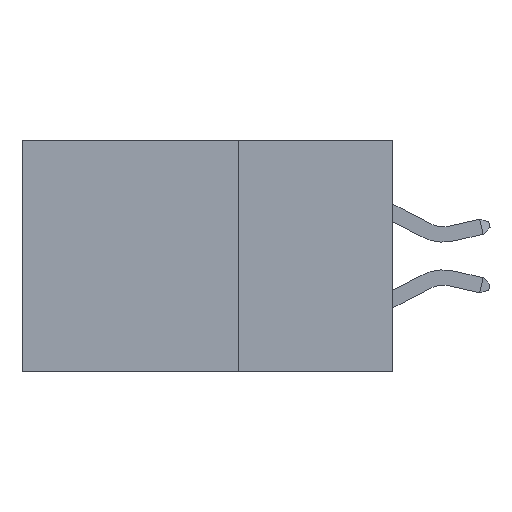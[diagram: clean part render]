
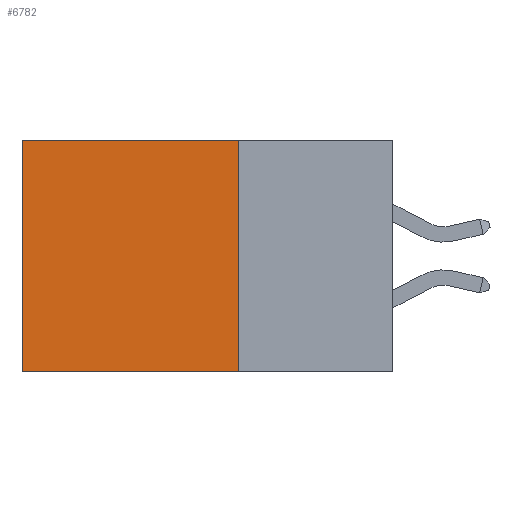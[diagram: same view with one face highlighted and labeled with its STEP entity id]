
A CAD part, left-side view. The second image highlights one B-rep face of the part: STEP entity #6782.
In plain terms, the highlighted planar face has unit normal (-1, 0, 0).
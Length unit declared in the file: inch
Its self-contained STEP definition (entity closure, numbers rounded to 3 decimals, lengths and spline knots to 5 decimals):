
#1126 = LINE ( 'NONE', #19039, #11063 ) ;
#1216 = EDGE_CURVE ( 'NONE', #10784, #21238, #11358, .T. ) ;
#1342 = VERTEX_POINT ( 'NONE', #4020 ) ;
#2004 = CARTESIAN_POINT ( 'NONE',  ( 0.2875, 0.25, -0.375 ) ) ;
#2983 = AXIS2_PLACEMENT_3D ( 'NONE', #11128, #14328, #4358 ) ;
#3239 = CARTESIAN_POINT ( 'NONE',  ( 0.2875, 0.25, 0. ) ) ;
#4020 = CARTESIAN_POINT ( 'NONE',  ( 0.2875, 0.25, 0. ) ) ;
#4358 = DIRECTION ( 'NONE',  ( 0., 0., -1. ) ) ;
#5771 = PLANE ( 'NONE',  #2983 ) ;
#6770 = VECTOR ( 'NONE', #12185, 39.37008 ) ;
#6782 = ADVANCED_FACE ( 'NONE', ( #12135 ), #5771, .F. ) ;
#7370 = DIRECTION ( 'NONE',  ( 0., 0., -1. ) ) ;
#7526 = CARTESIAN_POINT ( 'NONE',  ( 0.2875, 0.6, -0.375 ) ) ;
#10471 = DIRECTION ( 'NONE',  ( 0., 0., -1. ) ) ;
#10784 = VERTEX_POINT ( 'NONE', #16491 ) ;
#11063 = VECTOR ( 'NONE', #10471, 39.37008 ) ;
#11128 = CARTESIAN_POINT ( 'NONE',  ( 0.2875, 0.25, -0.375 ) ) ;
#11353 = ORIENTED_EDGE ( 'NONE', *, *, #21255, .F. ) ;
#11358 = LINE ( 'NONE', #2004, #6770 ) ;
#11375 = ORIENTED_EDGE ( 'NONE', *, *, #1216, .F. ) ;
#11800 = DIRECTION ( 'NONE',  ( 0., 1., 0. ) ) ;
#12135 = FACE_OUTER_BOUND ( 'NONE', #14568, .T. ) ;
#12185 = DIRECTION ( 'NONE',  ( 0., 1., 0. ) ) ;
#12885 = ORIENTED_EDGE ( 'NONE', *, *, #21916, .T. ) ;
#12985 = CARTESIAN_POINT ( 'NONE',  ( 0.2875, 0.6, 0. ) ) ;
#14328 = DIRECTION ( 'NONE',  ( 1., 0., 0. ) ) ;
#14568 = EDGE_LOOP ( 'NONE', ( #18636, #11375, #11353, #12885 ) ) ;
#14667 = LINE ( 'NONE', #15815, #19743 ) ;
#15815 = CARTESIAN_POINT ( 'NONE',  ( 0.2875, 0.25, -0.375 ) ) ;
#16255 = VERTEX_POINT ( 'NONE', #12985 ) ;
#16491 = CARTESIAN_POINT ( 'NONE',  ( 0.2875, 0.25, -0.375 ) ) ;
#18636 = ORIENTED_EDGE ( 'NONE', *, *, #19121, .T. ) ;
#19039 = CARTESIAN_POINT ( 'NONE',  ( 0.2875, 0.6, -0.375 ) ) ;
#19121 = EDGE_CURVE ( 'NONE', #16255, #21238, #1126, .T. ) ;
#19194 = VECTOR ( 'NONE', #11800, 39.37008 ) ;
#19719 = LINE ( 'NONE', #3239, #19194 ) ;
#19743 = VECTOR ( 'NONE', #7370, 39.37008 ) ;
#21238 = VERTEX_POINT ( 'NONE', #7526 ) ;
#21255 = EDGE_CURVE ( 'NONE', #1342, #10784, #14667, .T. ) ;
#21916 = EDGE_CURVE ( 'NONE', #1342, #16255, #19719, .T. ) ;
